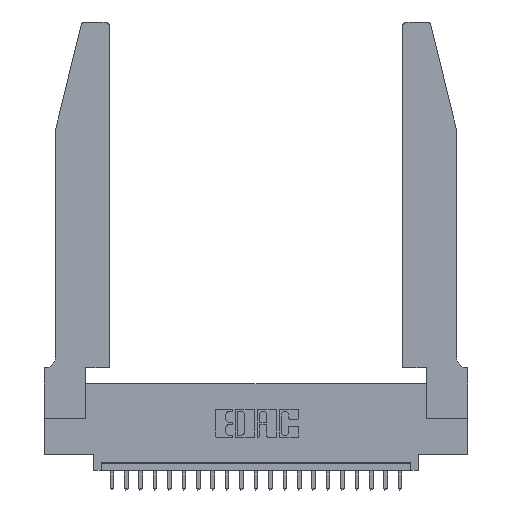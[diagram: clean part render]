
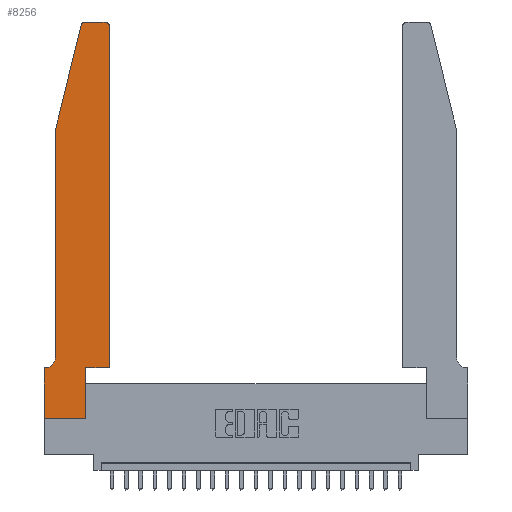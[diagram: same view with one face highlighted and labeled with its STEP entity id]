
A CAD part, top view. The second image highlights one B-rep face of the part: STEP entity #8256.
In plain terms, the highlighted planar face has unit normal (0, 0, 1).
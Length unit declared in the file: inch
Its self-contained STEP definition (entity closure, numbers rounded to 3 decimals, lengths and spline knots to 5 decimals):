
#349 = ORIENTED_EDGE ( 'NONE', *, *, #2489, .T. ) ;
#515 = DIRECTION ( 'NONE',  ( 0., 0., 1. ) ) ;
#790 = CARTESIAN_POINT ( 'NONE',  ( 0., 0.35, 0.37 ) ) ;
#822 = ORIENTED_EDGE ( 'NONE', *, *, #11899, .T. ) ;
#825 = CARTESIAN_POINT ( 'NONE',  ( 0.25487, 2.72718, 0.37 ) ) ;
#971 = ORIENTED_EDGE ( 'NONE', *, *, #5076, .T. ) ;
#1000 = LINE ( 'NONE', #9009, #2393 ) ;
#1176 = ORIENTED_EDGE ( 'NONE', *, *, #17347, .T. ) ;
#1395 = LINE ( 'NONE', #22499, #5090 ) ;
#1593 = DIRECTION ( 'NONE',  ( -1., 0., 0. ) ) ;
#2213 = LINE ( 'NONE', #11780, #5878 ) ;
#2393 = VECTOR ( 'NONE', #10853, 39.37008 ) ;
#2489 = EDGE_CURVE ( 'NONE', #20799, #11847, #2213, .T. ) ;
#2511 = VECTOR ( 'NONE', #13019, 39.37008 ) ;
#3059 = CARTESIAN_POINT ( 'NONE',  ( 0.0055, 0.35, 0.37 ) ) ;
#3322 = VERTEX_POINT ( 'NONE', #18006 ) ;
#3883 = CARTESIAN_POINT ( 'NONE',  ( 0., 0., 0.37 ) ) ;
#3957 = VECTOR ( 'NONE', #20368, 39.37008 ) ;
#4453 = DIRECTION ( 'NONE',  ( 1., 0., 0. ) ) ;
#4510 = VERTEX_POINT ( 'NONE', #11522 ) ;
#4579 = EDGE_CURVE ( 'NONE', #14522, #7386, #19564, .T. ) ;
#4716 = AXIS2_PLACEMENT_3D ( 'NONE', #15097, #18436, #18519 ) ;
#4791 = DIRECTION ( 'NONE',  ( -1., 0., 0. ) ) ;
#5027 = AXIS2_PLACEMENT_3D ( 'NONE', #11306, #515, #20449 ) ;
#5076 = EDGE_CURVE ( 'NONE', #7386, #12349, #20075, .T. ) ;
#5090 = VECTOR ( 'NONE', #4453, 39.37008 ) ;
#5420 = CARTESIAN_POINT ( 'NONE',  ( 0.4505, 2.72, 0.37 ) ) ;
#5581 = LINE ( 'NONE', #9959, #17769 ) ;
#5834 = ORIENTED_EDGE ( 'NONE', *, *, #10117, .T. ) ;
#5878 = VECTOR ( 'NONE', #15185, 39.37008 ) ;
#6635 = CARTESIAN_POINT ( 'NONE',  ( 0.0055, 0.42, 0.37 ) ) ;
#6787 = EDGE_CURVE ( 'NONE', #12200, #17460, #18850, .T. ) ;
#7386 = VERTEX_POINT ( 'NONE', #790 ) ;
#7628 = CARTESIAN_POINT ( 'NONE',  ( 0.4505, 0.35, 0.37 ) ) ;
#7944 = VERTEX_POINT ( 'NONE', #23534 ) ;
#8256 = ADVANCED_FACE ( 'NONE', ( #19096 ), #9639, .T. ) ;
#8794 = DIRECTION ( 'NONE',  ( 0., 0., 1. ) ) ;
#9009 = CARTESIAN_POINT ( 'NONE',  ( 0.2865, 0.35, 0.37 ) ) ;
#9476 = ORIENTED_EDGE ( 'NONE', *, *, #4579, .T. ) ;
#9605 = LINE ( 'NONE', #18706, #3957 ) ;
#9639 = PLANE ( 'NONE',  #5027 ) ;
#9654 = AXIS2_PLACEMENT_3D ( 'NONE', #6635, #14983, #1593 ) ;
#9879 = VECTOR ( 'NONE', #4791, 39.37008 ) ;
#9959 = CARTESIAN_POINT ( 'NONE',  ( 0.2605, 2.75, 0.37 ) ) ;
#10096 = AXIS2_PLACEMENT_3D ( 'NONE', #21343, #8794, #21504 ) ;
#10101 = ORIENTED_EDGE ( 'NONE', *, *, #17816, .T. ) ;
#10117 = EDGE_CURVE ( 'NONE', #4510, #14522, #14455, .T. ) ;
#10853 = DIRECTION ( 'NONE',  ( 0., 1., 0. ) ) ;
#11306 = CARTESIAN_POINT ( 'NONE',  ( 0., 0.35, 0.37 ) ) ;
#11522 = CARTESIAN_POINT ( 'NONE',  ( 0.0755, 0.42, 0.37 ) ) ;
#11625 = DIRECTION ( 'NONE',  ( -1., 0., 0. ) ) ;
#11780 = CARTESIAN_POINT ( 'NONE',  ( 0.0755, 2., 0.37 ) ) ;
#11847 = VERTEX_POINT ( 'NONE', #18454 ) ;
#11899 = EDGE_CURVE ( 'NONE', #11847, #4510, #9605, .T. ) ;
#12200 = VERTEX_POINT ( 'NONE', #5420 ) ;
#12349 = VERTEX_POINT ( 'NONE', #3883 ) ;
#13019 = DIRECTION ( 'NONE',  ( 0., 1., 0. ) ) ;
#13042 = CARTESIAN_POINT ( 'NONE',  ( 0.284, 2.75, 0.37 ) ) ;
#13135 = ORIENTED_EDGE ( 'NONE', *, *, #22291, .T. ) ;
#13234 = EDGE_CURVE ( 'NONE', #17959, #3322, #14387, .T. ) ;
#13561 = ORIENTED_EDGE ( 'NONE', *, *, #6787, .T. ) ;
#14104 = VECTOR ( 'NONE', #20882, 39.37008 ) ;
#14142 = EDGE_CURVE ( 'NONE', #7944, #17959, #1000, .T. ) ;
#14387 = LINE ( 'NONE', #15467, #20351 ) ;
#14455 = CIRCLE ( 'NONE', #9654, 0.07 ) ;
#14522 = VERTEX_POINT ( 'NONE', #3059 ) ;
#14556 = CIRCLE ( 'NONE', #10096, 0.03 ) ;
#14983 = DIRECTION ( 'NONE',  ( 0., 0., -1. ) ) ;
#15097 = CARTESIAN_POINT ( 'NONE',  ( 0.4205, 2.72, 0.37 ) ) ;
#15185 = DIRECTION ( 'NONE',  ( -0.239, -0.971, 0. ) ) ;
#15308 = DIRECTION ( 'NONE',  ( 1., 0., 0. ) ) ;
#15467 = CARTESIAN_POINT ( 'NONE',  ( 0.4505, 0.35, 0.37 ) ) ;
#17285 = ORIENTED_EDGE ( 'NONE', *, *, #13234, .T. ) ;
#17347 = EDGE_CURVE ( 'NONE', #17460, #18365, #5581, .T. ) ;
#17460 = VERTEX_POINT ( 'NONE', #21324 ) ;
#17769 = VECTOR ( 'NONE', #11625, 39.37008 ) ;
#17816 = EDGE_CURVE ( 'NONE', #3322, #12200, #18156, .T. ) ;
#17959 = VERTEX_POINT ( 'NONE', #22822 ) ;
#18006 = CARTESIAN_POINT ( 'NONE',  ( 0.4505, 0.35, 0.37 ) ) ;
#18031 = EDGE_CURVE ( 'NONE', #12349, #7944, #1395, .T. ) ;
#18156 = LINE ( 'NONE', #7628, #2511 ) ;
#18365 = VERTEX_POINT ( 'NONE', #13042 ) ;
#18436 = DIRECTION ( 'NONE',  ( 0., 0., 1. ) ) ;
#18454 = CARTESIAN_POINT ( 'NONE',  ( 0.0755, 2., 0.37 ) ) ;
#18519 = DIRECTION ( 'NONE',  ( 1., 0., 0. ) ) ;
#18706 = CARTESIAN_POINT ( 'NONE',  ( 0.0755, 2., 0.37 ) ) ;
#18850 = CIRCLE ( 'NONE', #4716, 0.03 ) ;
#19070 = CARTESIAN_POINT ( 'NONE',  ( 0., 0., 0.37 ) ) ;
#19096 = FACE_OUTER_BOUND ( 'NONE', #20583, .T. ) ;
#19380 = ORIENTED_EDGE ( 'NONE', *, *, #18031, .T. ) ;
#19564 = LINE ( 'NONE', #20975, #9879 ) ;
#19970 = ORIENTED_EDGE ( 'NONE', *, *, #14142, .T. ) ;
#20075 = LINE ( 'NONE', #19070, #14104 ) ;
#20351 = VECTOR ( 'NONE', #15308, 39.37008 ) ;
#20368 = DIRECTION ( 'NONE',  ( 0., -1., 0. ) ) ;
#20449 = DIRECTION ( 'NONE',  ( 1., 0., 0. ) ) ;
#20583 = EDGE_LOOP ( 'NONE', ( #1176, #13135, #349, #822, #5834, #9476, #971, #19380, #19970, #17285, #10101, #13561 ) ) ;
#20799 = VERTEX_POINT ( 'NONE', #825 ) ;
#20882 = DIRECTION ( 'NONE',  ( 0., -1., 0. ) ) ;
#20975 = CARTESIAN_POINT ( 'NONE',  ( 0.0755, 0.35, 0.37 ) ) ;
#21324 = CARTESIAN_POINT ( 'NONE',  ( 0.4205, 2.75, 0.37 ) ) ;
#21343 = CARTESIAN_POINT ( 'NONE',  ( 0.284, 2.72, 0.37 ) ) ;
#21504 = DIRECTION ( 'NONE',  ( 1., 0., 0. ) ) ;
#22291 = EDGE_CURVE ( 'NONE', #18365, #20799, #14556, .T. ) ;
#22499 = CARTESIAN_POINT ( 'NONE',  ( 0., 0., 0.37 ) ) ;
#22822 = CARTESIAN_POINT ( 'NONE',  ( 0.2865, 0.35, 0.37 ) ) ;
#23534 = CARTESIAN_POINT ( 'NONE',  ( 0.2865, 0., 0.37 ) ) ;
